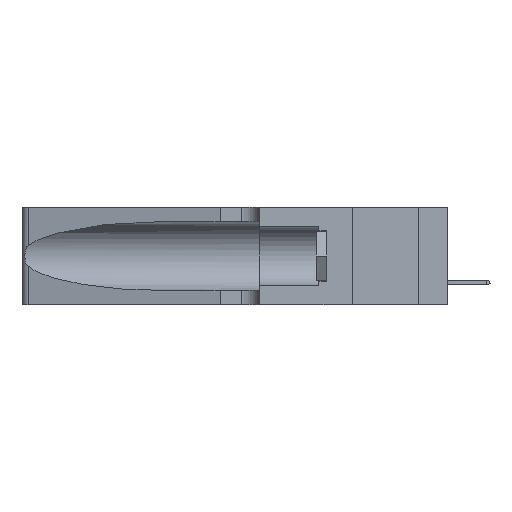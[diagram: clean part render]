
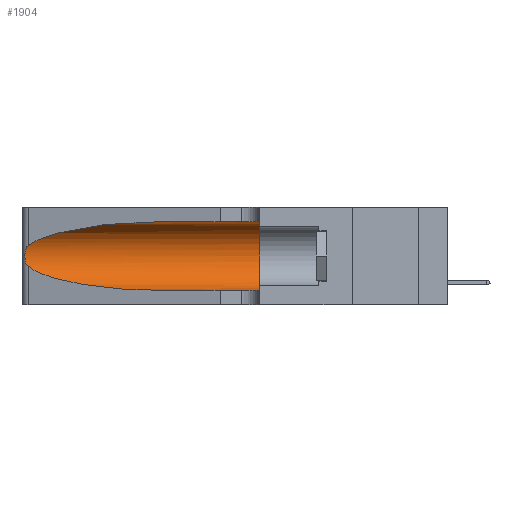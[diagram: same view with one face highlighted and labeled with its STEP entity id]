
A CAD part, left-side view. The second image highlights one B-rep face of the part: STEP entity #1904.
In plain terms, the highlighted cylindrical face has radius 3.308 mm (diameter 6.617 mm), a partial arc.
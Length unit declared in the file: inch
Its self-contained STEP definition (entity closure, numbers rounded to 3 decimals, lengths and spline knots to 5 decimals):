
#541 = EDGE_CURVE ( 'NONE', #12800, #11731, #20903, .T. ) ;
#683 = VERTEX_POINT ( 'NONE', #7401 ) ;
#1217 = CARTESIAN_POINT ( 'NONE',  ( 0.25856, 1.23593, 0.16098 ) ) ;
#1904 = ADVANCED_FACE ( 'NONE', ( #2011 ), #21517, .F. ) ;
#2011 = FACE_OUTER_BOUND ( 'NONE', #13683, .T. ) ;
#2385 = CARTESIAN_POINT ( 'NONE',  ( 0.1305, 1.61858, 0.185 ) ) ;
#2407 = CARTESIAN_POINT ( 'NONE',  ( 0.2373, 1.15595, 0.08982 ) ) ;
#2938 = CARTESIAN_POINT ( 'NONE',  ( 0.25639, 1.23184, 0.21858 ) ) ;
#3025 = CARTESIAN_POINT ( 'NONE',  ( 0.1305, 0.72297, 0.31525 ) ) ;
#3179 = CARTESIAN_POINT ( 'NONE',  ( 0.25787, 1.23484, 0.2124 ) ) ;
#3262 = CARTESIAN_POINT ( 'NONE',  ( 0.26017, 1.23833, 0.17102 ) ) ;
#3275 = CARTESIAN_POINT ( 'NONE',  ( 0.1305, 1.61858, 0.31525 ) ) ;
#4341 = ORIENTED_EDGE ( 'NONE', *, *, #9071, .T. ) ;
#4407 = CARTESIAN_POINT ( 'NONE',  ( 0.18966, 0.96281, 0.31525 ) ) ;
#4982 = DIRECTION ( 'NONE',  ( 0., 0., -1. ) ) ;
#5525 = EDGE_CURVE ( 'NONE', #11731, #10423, #13438, .T. ) ;
#5872 = CARTESIAN_POINT ( 'NONE',  ( 0.1305, 0.72297, 0.31525 ) ) ;
#5875 = VECTOR ( 'NONE', #16429, 39.37008 ) ;
#6631 = CIRCLE ( 'NONE', #20471, 0.13025 ) ;
#6633 = DIRECTION ( 'NONE',  ( 0., -1., 0. ) ) ;
#6836 = CARTESIAN_POINT ( 'NONE',  ( 0.25854, 1.2359, 0.20912 ) ) ;
#7401 = CARTESIAN_POINT ( 'NONE',  ( 0.1305, 0.35, 0.05475 ) ) ;
#7928 = CARTESIAN_POINT ( 'NONE',  ( 0.18966, 0.96281, 0.05475 ) ) ;
#7955 = CARTESIAN_POINT ( 'NONE',  ( 0.25487, 1.22718, 0.22369 ) ) ;
#8101 = CARTESIAN_POINT ( 'NONE',  ( 0.1305, 0.72297, 0.05475 ) ) ;
#8618 = CARTESIAN_POINT ( 'NONE',  ( 0.25487, 1.22718, 0.22369 ) ) ;
#9071 = EDGE_CURVE ( 'NONE', #10423, #15205, #19109, .T. ) ;
#9904 = CARTESIAN_POINT ( 'NONE',  ( 0.1305, 0.35, 0.31525 ) ) ;
#10423 = VERTEX_POINT ( 'NONE', #20845 ) ;
#10440 = CARTESIAN_POINT ( 'NONE',  ( 0.25487, 1.22718, 0.14631 ) ) ;
#11223 = AXIS2_PLACEMENT_3D ( 'NONE', #2385, #6633, #4982 ) ;
#11276 = DIRECTION ( 'NONE',  ( 0., 1., 0. ) ) ;
#11526 = VERTEX_POINT ( 'NONE', #9904 ) ;
#11627 = CARTESIAN_POINT ( 'NONE',  ( 0.25487, 1.22718, 0.22369 ) ) ;
#11731 = VERTEX_POINT ( 'NONE', #11627 ) ;
#12368 = CARTESIAN_POINT ( 'NONE',  ( 0.26075, 1.23896, 0.19203 ) ) ;
#12800 = VERTEX_POINT ( 'NONE', #5872 ) ;
#13438 = B_SPLINE_CURVE_WITH_KNOTS ( 'NONE', 3,
 ( #8618, #14060, #2938, #3179, #6836, #21596, #12368, #19808, #3262, #1217, #23590, #15939, #19639, #10440 ),
 .UNSPECIFIED., .F., .F.,
 ( 4, 2, 2, 2, 2, 2, 4 ),
 ( 0., 0.00027, 0.00053, 0.00107, 0.0016, 0.00187, 0.00214 ),
 .UNSPECIFIED. ) ;
#13520 = CARTESIAN_POINT ( 'NONE',  ( 0.25487, 1.22718, 0.14631 ) ) ;
#13579 = CARTESIAN_POINT ( 'NONE',  ( 0.1305, 1.61858, 0.05475 ) ) ;
#13683 = EDGE_LOOP ( 'NONE', ( #20771, #14279, #4341, #21427, #16811, #22416 ) ) ;
#14060 = CARTESIAN_POINT ( 'NONE',  ( 0.25555, 1.22994, 0.2215 ) ) ;
#14279 = ORIENTED_EDGE ( 'NONE', *, *, #5525, .T. ) ;
#14917 = DIRECTION ( 'NONE',  ( 0., 0., 1. ) ) ;
#15181 = CARTESIAN_POINT ( 'NONE',  ( 0.1305, 0.72297, 0.05475 ) ) ;
#15205 = VERTEX_POINT ( 'NONE', #15181 ) ;
#15632 = LINE ( 'NONE', #13579, #20250 ) ;
#15939 = CARTESIAN_POINT ( 'NONE',  ( 0.25639, 1.23186, 0.15144 ) ) ;
#16429 = DIRECTION ( 'NONE',  ( 0., -1., 0. ) ) ;
#16811 = ORIENTED_EDGE ( 'NONE', *, *, #21785, .F. ) ;
#17408 = CARTESIAN_POINT ( 'NONE',  ( 0.2373, 1.15595, 0.28018 ) ) ;
#17435 = DIRECTION ( 'NONE',  ( 0., -1., 0. ) ) ;
#18361 = LINE ( 'NONE', #3275, #5875 ) ;
#18472 = CARTESIAN_POINT ( 'NONE',  ( 0.1305, 0.35, 0.185 ) ) ;
#19109 =( BOUNDED_CURVE ( )  B_SPLINE_CURVE ( 3, ( #13520, #2407, #7928, #8101 ),
 .UNSPECIFIED., .F., .T. ) 
 B_SPLINE_CURVE_WITH_KNOTS ( ( 4, 4 ),
 ( 3.44316, 4.71239 ),
 .UNSPECIFIED. ) 
 CURVE ( )  GEOMETRIC_REPRESENTATION_ITEM ( )  RATIONAL_B_SPLINE_CURVE ( ( 1., 0.87, 0.87, 1. ) ) 
 REPRESENTATION_ITEM ( '' )  );
#19307 = EDGE_CURVE ( 'NONE', #12800, #11526, #18361, .T. ) ;
#19639 = CARTESIAN_POINT ( 'NONE',  ( 0.25555, 1.22993, 0.14849 ) ) ;
#19808 = CARTESIAN_POINT ( 'NONE',  ( 0.26075, 1.23896, 0.178 ) ) ;
#20250 = VECTOR ( 'NONE', #17435, 39.37008 ) ;
#20471 = AXIS2_PLACEMENT_3D ( 'NONE', #18472, #11276, #14917 ) ;
#20771 = ORIENTED_EDGE ( 'NONE', *, *, #541, .T. ) ;
#20845 = CARTESIAN_POINT ( 'NONE',  ( 0.25487, 1.22718, 0.14631 ) ) ;
#20903 =( BOUNDED_CURVE ( )  B_SPLINE_CURVE ( 3, ( #3025, #4407, #17408, #7955 ),
 .UNSPECIFIED., .F., .F. ) 
 B_SPLINE_CURVE_WITH_KNOTS ( ( 4, 4 ),
 ( 1.5708, 2.84003 ),
 .UNSPECIFIED. ) 
 CURVE ( )  GEOMETRIC_REPRESENTATION_ITEM ( )  RATIONAL_B_SPLINE_CURVE ( ( 1., 0.87, 0.87, 1. ) ) 
 REPRESENTATION_ITEM ( '' )  );
#21427 = ORIENTED_EDGE ( 'NONE', *, *, #22010, .T. ) ;
#21517 = CYLINDRICAL_SURFACE ( 'NONE', #11223, 0.13025 ) ;
#21596 = CARTESIAN_POINT ( 'NONE',  ( 0.26018, 1.23835, 0.19895 ) ) ;
#21785 = EDGE_CURVE ( 'NONE', #11526, #683, #6631, .T. ) ;
#22010 = EDGE_CURVE ( 'NONE', #15205, #683, #15632, .T. ) ;
#22416 = ORIENTED_EDGE ( 'NONE', *, *, #19307, .F. ) ;
#23590 = CARTESIAN_POINT ( 'NONE',  ( 0.25789, 1.23486, 0.15765 ) ) ;
